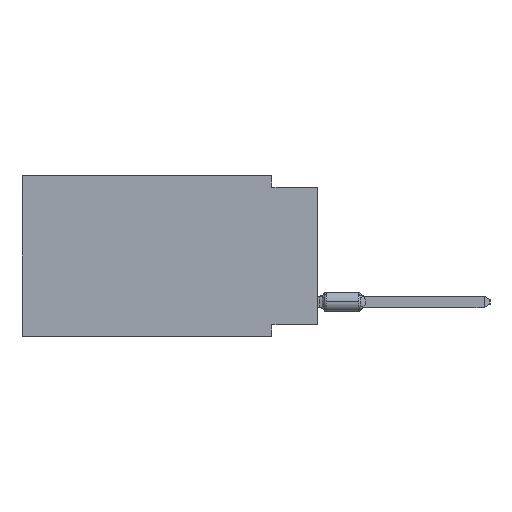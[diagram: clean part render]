
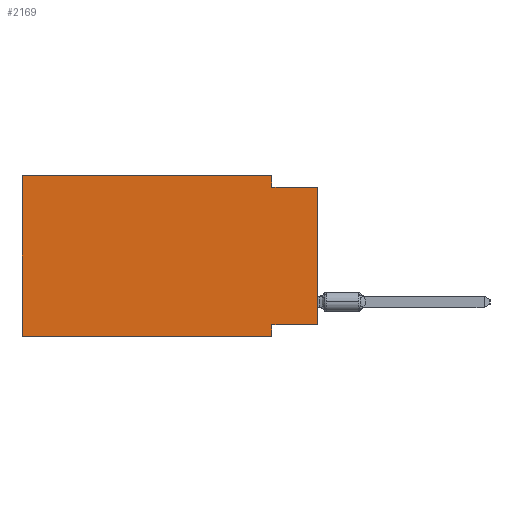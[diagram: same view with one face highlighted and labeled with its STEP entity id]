
A CAD part, left-side view. The second image highlights one B-rep face of the part: STEP entity #2169.
In plain terms, the highlighted planar face has unit normal (-1, 0, 0).
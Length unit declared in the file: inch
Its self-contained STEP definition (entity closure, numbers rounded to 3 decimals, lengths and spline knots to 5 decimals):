
#769 = EDGE_CURVE ( 'NONE', #11263, #39884, #6998, .T. ) ;
#924 = CARTESIAN_POINT ( 'NONE',  ( 0., 0.645, 0. ) ) ;
#1332 = EDGE_CURVE ( 'NONE', #28068, #15267, #18965, .T. ) ;
#1761 = VECTOR ( 'NONE', #36413, 39.37008 ) ;
#1780 = DIRECTION ( 'NONE',  ( 0., -1., 0. ) ) ;
#1908 = ORIENTED_EDGE ( 'NONE', *, *, #37441, .F. ) ;
#2169 = ADVANCED_FACE ( 'NONE', ( #18599 ), #32760, .F. ) ;
#2957 = EDGE_CURVE ( 'NONE', #30172, #8282, #15290, .T. ) ;
#3014 = EDGE_CURVE ( 'NONE', #30172, #6638, #45019, .T. ) ;
#3754 = LINE ( 'NONE', #17937, #13922 ) ;
#4410 = ORIENTED_EDGE ( 'NONE', *, *, #769, .F. ) ;
#5420 = DIRECTION ( 'NONE',  ( 0., -1., 0. ) ) ;
#5506 = ORIENTED_EDGE ( 'NONE', *, *, #3014, .T. ) ;
#6638 = VERTEX_POINT ( 'NONE', #35516 ) ;
#6998 = LINE ( 'NONE', #7221, #24818 ) ;
#7221 = CARTESIAN_POINT ( 'NONE',  ( 0., 0., -0.325 ) ) ;
#8282 = VERTEX_POINT ( 'NONE', #30157 ) ;
#8313 = CARTESIAN_POINT ( 'NONE',  ( 0., 0.645, 0. ) ) ;
#11263 = VERTEX_POINT ( 'NONE', #13116 ) ;
#12948 = CARTESIAN_POINT ( 'NONE',  ( 0., 0., -0.025 ) ) ;
#13116 = CARTESIAN_POINT ( 'NONE',  ( 0., 0., -0.325 ) ) ;
#13485 = ORIENTED_EDGE ( 'NONE', *, *, #1332, .F. ) ;
#13922 = VECTOR ( 'NONE', #21834, 39.37008 ) ;
#15107 = DIRECTION ( 'NONE',  ( 1., 0., 0. ) ) ;
#15267 = VERTEX_POINT ( 'NONE', #20379 ) ;
#15290 = LINE ( 'NONE', #8313, #35318 ) ;
#15765 = VECTOR ( 'NONE', #5420, 39.37008 ) ;
#15767 = LINE ( 'NONE', #40615, #37563 ) ;
#16945 = CARTESIAN_POINT ( 'NONE',  ( 0., 0.1, 0. ) ) ;
#17550 = EDGE_CURVE ( 'NONE', #39884, #6638, #45786, .T. ) ;
#17937 = CARTESIAN_POINT ( 'NONE',  ( 0., 0., 0. ) ) ;
#18413 = EDGE_CURVE ( 'NONE', #15267, #41507, #15767, .T. ) ;
#18599 = FACE_OUTER_BOUND ( 'NONE', #45225, .T. ) ;
#18965 = LINE ( 'NONE', #21771, #1761 ) ;
#20379 = CARTESIAN_POINT ( 'NONE',  ( 0., 0.1, -0.025 ) ) ;
#21771 = CARTESIAN_POINT ( 'NONE',  ( 0., 0.1, 0. ) ) ;
#21807 = ORIENTED_EDGE ( 'NONE', *, *, #2957, .F. ) ;
#21834 = DIRECTION ( 'NONE',  ( 0., 0., 1. ) ) ;
#22360 = EDGE_CURVE ( 'NONE', #11263, #41507, #3754, .T. ) ;
#22809 = ORIENTED_EDGE ( 'NONE', *, *, #17550, .F. ) ;
#23366 = VECTOR ( 'NONE', #42303, 39.37008 ) ;
#24149 = VECTOR ( 'NONE', #1780, 39.37008 ) ;
#24818 = VECTOR ( 'NONE', #28782, 39.37008 ) ;
#25949 = DIRECTION ( 'NONE',  ( 0., -1., 0. ) ) ;
#28068 = VERTEX_POINT ( 'NONE', #16945 ) ;
#28076 = CARTESIAN_POINT ( 'NONE',  ( 0., 0.645, -0.35 ) ) ;
#28106 = CARTESIAN_POINT ( 'NONE',  ( 0., 0.1, -0.35 ) ) ;
#28782 = DIRECTION ( 'NONE',  ( 0., 1., 0. ) ) ;
#29247 = DIRECTION ( 'NONE',  ( 0., 0., -1. ) ) ;
#30157 = CARTESIAN_POINT ( 'NONE',  ( 0., 0.645, 0. ) ) ;
#30172 = VERTEX_POINT ( 'NONE', #28076 ) ;
#30599 = CARTESIAN_POINT ( 'NONE',  ( 0., 0.645, -0.35 ) ) ;
#32234 = ORIENTED_EDGE ( 'NONE', *, *, #18413, .F. ) ;
#32760 = PLANE ( 'NONE',  #44029 ) ;
#35318 = VECTOR ( 'NONE', #38049, 39.37008 ) ;
#35516 = CARTESIAN_POINT ( 'NONE',  ( 0., 0.1, -0.35 ) ) ;
#36413 = DIRECTION ( 'NONE',  ( 0., 0., -1. ) ) ;
#37441 = EDGE_CURVE ( 'NONE', #8282, #28068, #39209, .T. ) ;
#37563 = VECTOR ( 'NONE', #25949, 39.37008 ) ;
#37946 = CARTESIAN_POINT ( 'NONE',  ( 0., 0.645, 0. ) ) ;
#38049 = DIRECTION ( 'NONE',  ( 0., 0., 1. ) ) ;
#39209 = LINE ( 'NONE', #37946, #15765 ) ;
#39884 = VERTEX_POINT ( 'NONE', #45652 ) ;
#40615 = CARTESIAN_POINT ( 'NONE',  ( 0., 0., -0.025 ) ) ;
#41507 = VERTEX_POINT ( 'NONE', #12948 ) ;
#42303 = DIRECTION ( 'NONE',  ( 0., 0., -1. ) ) ;
#43318 = ORIENTED_EDGE ( 'NONE', *, *, #22360, .T. ) ;
#44029 = AXIS2_PLACEMENT_3D ( 'NONE', #924, #15107, #29247 ) ;
#45019 = LINE ( 'NONE', #30599, #24149 ) ;
#45225 = EDGE_LOOP ( 'NONE', ( #43318, #32234, #13485, #1908, #21807, #5506, #22809, #4410 ) ) ;
#45652 = CARTESIAN_POINT ( 'NONE',  ( 0., 0.1, -0.325 ) ) ;
#45786 = LINE ( 'NONE', #28106, #23366 ) ;
